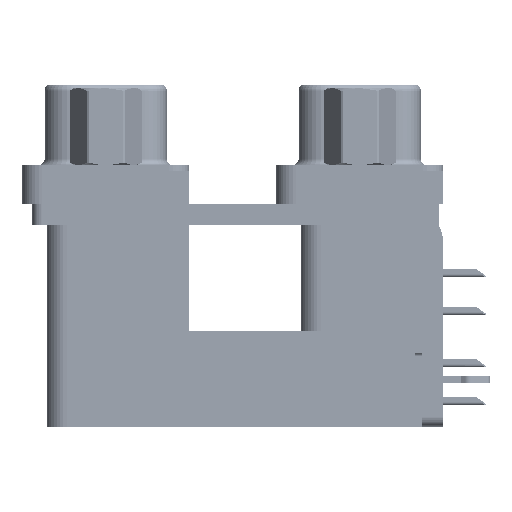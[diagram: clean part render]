
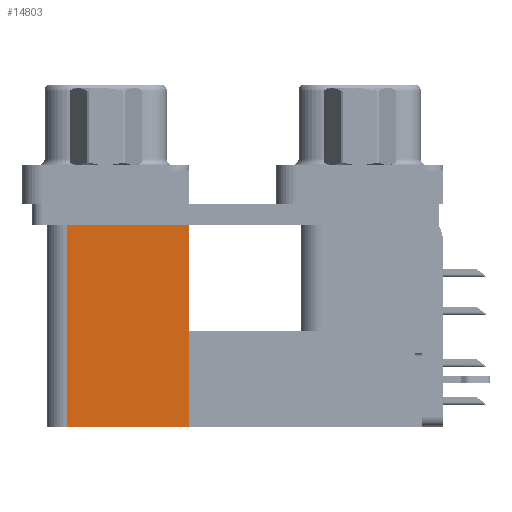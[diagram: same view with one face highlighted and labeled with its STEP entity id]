
A CAD part, left-side view. The second image highlights one B-rep face of the part: STEP entity #14803.
In plain terms, the highlighted planar face has unit normal (-1, 0, 0).
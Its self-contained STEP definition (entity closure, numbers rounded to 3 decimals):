
#1692 = DIRECTION ( 'NONE',  ( 0., 1., 0. ) ) ;
#1910 = CARTESIAN_POINT ( 'NONE',  ( 3.79, 12.775, -2.5 ) ) ;
#5617 = VECTOR ( 'NONE', #10857, 1000. ) ;
#6818 = EDGE_CURVE ( 'NONE', #28628, #33122, #52420, .T. ) ;
#9326 = LINE ( 'NONE', #22742, #52619 ) ;
#10340 = EDGE_CURVE ( 'NONE', #44765, #47573, #52020, .T. ) ;
#10857 = DIRECTION ( 'NONE',  ( 0., 0., 1. ) ) ;
#12273 = DIRECTION ( 'NONE',  ( 1., 0., 0. ) ) ;
#12795 = CARTESIAN_POINT ( 'NONE',  ( 3.79, 21.975, -19.2 ) ) ;
#14803 = ADVANCED_FACE ( 'NONE', ( #52180 ), #20145, .F. ) ;
#20145 = PLANE ( 'NONE',  #31921 ) ;
#20735 = EDGE_CURVE ( 'NONE', #47573, #33122, #30408, .T. ) ;
#22742 = CARTESIAN_POINT ( 'NONE',  ( 3.79, 12.775, -19.2 ) ) ;
#23186 = VECTOR ( 'NONE', #39452, 1000. ) ;
#27926 = ORIENTED_EDGE ( 'NONE', *, *, #6818, .F. ) ;
#28628 = VERTEX_POINT ( 'NONE', #47149 ) ;
#29885 = CARTESIAN_POINT ( 'NONE',  ( 3.79, 12.775, -19.2 ) ) ;
#30408 = LINE ( 'NONE', #48168, #23186 ) ;
#31921 = AXIS2_PLACEMENT_3D ( 'NONE', #51601, #12273, #46941 ) ;
#32739 = ORIENTED_EDGE ( 'NONE', *, *, #20735, .T. ) ;
#33122 = VERTEX_POINT ( 'NONE', #52587 ) ;
#38753 = DIRECTION ( 'NONE',  ( 0., 0., 1. ) ) ;
#39452 = DIRECTION ( 'NONE',  ( 0., 1., 0. ) ) ;
#40822 = EDGE_LOOP ( 'NONE', ( #32739, #27926, #49954, #47708 ) ) ;
#44765 = VERTEX_POINT ( 'NONE', #54867 ) ;
#46049 = VECTOR ( 'NONE', #38753, 1000. ) ;
#46941 = DIRECTION ( 'NONE',  ( 0., 0., -1. ) ) ;
#47149 = CARTESIAN_POINT ( 'NONE',  ( 3.79, 21.975, -19.2 ) ) ;
#47573 = VERTEX_POINT ( 'NONE', #1910 ) ;
#47708 = ORIENTED_EDGE ( 'NONE', *, *, #10340, .T. ) ;
#48168 = CARTESIAN_POINT ( 'NONE',  ( 3.79, 12.775, -2.5 ) ) ;
#49954 = ORIENTED_EDGE ( 'NONE', *, *, #53458, .F. ) ;
#51601 = CARTESIAN_POINT ( 'NONE',  ( 3.79, 12.775, -19.2 ) ) ;
#52020 = LINE ( 'NONE', #29885, #5617 ) ;
#52180 = FACE_OUTER_BOUND ( 'NONE', #40822, .T. ) ;
#52420 = LINE ( 'NONE', #12795, #46049 ) ;
#52587 = CARTESIAN_POINT ( 'NONE',  ( 3.79, 21.975, -2.5 ) ) ;
#52619 = VECTOR ( 'NONE', #1692, 1000. ) ;
#53458 = EDGE_CURVE ( 'NONE', #44765, #28628, #9326, .T. ) ;
#54867 = CARTESIAN_POINT ( 'NONE',  ( 3.79, 12.775, -19.2 ) ) ;
